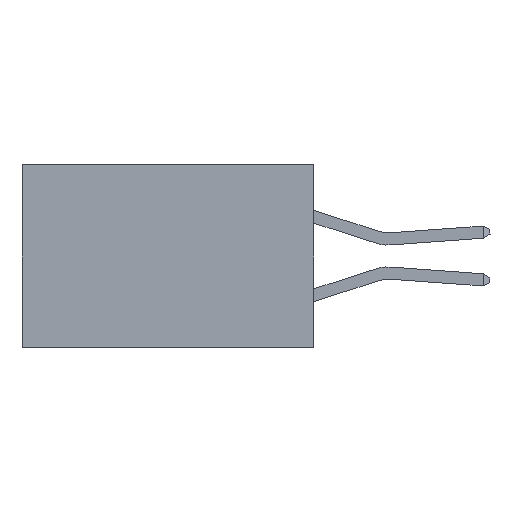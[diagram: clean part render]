
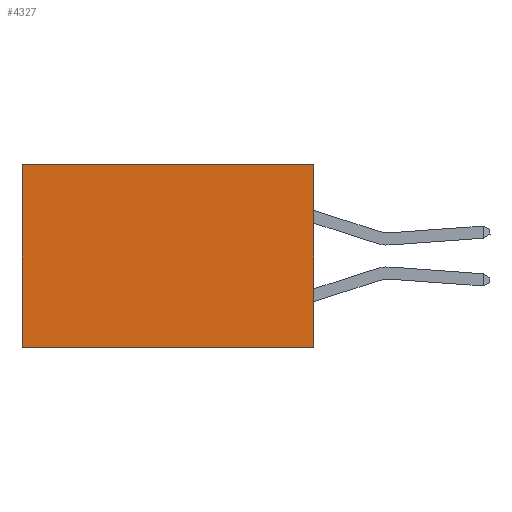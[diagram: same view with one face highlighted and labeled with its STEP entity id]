
A CAD part, left-side view. The second image highlights one B-rep face of the part: STEP entity #4327.
In plain terms, the highlighted planar face has unit normal (-1, 0, 0).
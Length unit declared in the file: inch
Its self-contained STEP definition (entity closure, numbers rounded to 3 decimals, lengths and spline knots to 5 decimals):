
#518 = ORIENTED_EDGE ( 'NONE', *, *, #2243, .F. ) ;
#761 = CARTESIAN_POINT ( 'NONE',  ( 0.2875, 0., 0. ) ) ;
#906 = VECTOR ( 'NONE', #2221, 39.37008 ) ;
#1702 = CARTESIAN_POINT ( 'NONE',  ( 0.2875, 0.6, -0.375 ) ) ;
#1955 = VERTEX_POINT ( 'NONE', #761 ) ;
#2023 = DIRECTION ( 'NONE',  ( 1., 0., 0. ) ) ;
#2221 = DIRECTION ( 'NONE',  ( 0., 1., 0. ) ) ;
#2243 = EDGE_CURVE ( 'NONE', #1955, #10612, #12016, .T. ) ;
#2283 = VECTOR ( 'NONE', #5648, 39.37008 ) ;
#2723 = CARTESIAN_POINT ( 'NONE',  ( 0.2875, 0., -0.375 ) ) ;
#2790 = LINE ( 'NONE', #1702, #9710 ) ;
#2843 = FACE_OUTER_BOUND ( 'NONE', #8363, .T. ) ;
#3217 = VERTEX_POINT ( 'NONE', #9706 ) ;
#4327 = ADVANCED_FACE ( 'NONE', ( #2843 ), #12202, .F. ) ;
#5486 = CARTESIAN_POINT ( 'NONE',  ( 0.2875, 0., -0.375 ) ) ;
#5648 = DIRECTION ( 'NONE',  ( 0., 0., -1. ) ) ;
#5686 = VECTOR ( 'NONE', #9636, 39.37008 ) ;
#5926 = DIRECTION ( 'NONE',  ( 0., 0., -1. ) ) ;
#5945 = EDGE_CURVE ( 'NONE', #10612, #3217, #12728, .T. ) ;
#7662 = AXIS2_PLACEMENT_3D ( 'NONE', #7963, #2023, #13359 ) ;
#7963 = CARTESIAN_POINT ( 'NONE',  ( 0.2875, 0., -0.375 ) ) ;
#8363 = EDGE_LOOP ( 'NONE', ( #8835, #11467, #518, #12662 ) ) ;
#8835 = ORIENTED_EDGE ( 'NONE', *, *, #9856, .T. ) ;
#8996 = EDGE_CURVE ( 'NONE', #1955, #11040, #9429, .T. ) ;
#9364 = CARTESIAN_POINT ( 'NONE',  ( 0.2875, 0., 0. ) ) ;
#9429 = LINE ( 'NONE', #9364, #5686 ) ;
#9636 = DIRECTION ( 'NONE',  ( 0., 1., 0. ) ) ;
#9706 = CARTESIAN_POINT ( 'NONE',  ( 0.2875, 0.6, -0.375 ) ) ;
#9710 = VECTOR ( 'NONE', #5926, 39.37008 ) ;
#9856 = EDGE_CURVE ( 'NONE', #11040, #3217, #2790, .T. ) ;
#10612 = VERTEX_POINT ( 'NONE', #13071 ) ;
#11040 = VERTEX_POINT ( 'NONE', #12619 ) ;
#11467 = ORIENTED_EDGE ( 'NONE', *, *, #5945, .F. ) ;
#12016 = LINE ( 'NONE', #2723, #2283 ) ;
#12202 = PLANE ( 'NONE',  #7662 ) ;
#12619 = CARTESIAN_POINT ( 'NONE',  ( 0.2875, 0.6, 0. ) ) ;
#12662 = ORIENTED_EDGE ( 'NONE', *, *, #8996, .T. ) ;
#12728 = LINE ( 'NONE', #5486, #906 ) ;
#13071 = CARTESIAN_POINT ( 'NONE',  ( 0.2875, 0., -0.375 ) ) ;
#13359 = DIRECTION ( 'NONE',  ( 0., 0., -1. ) ) ;
